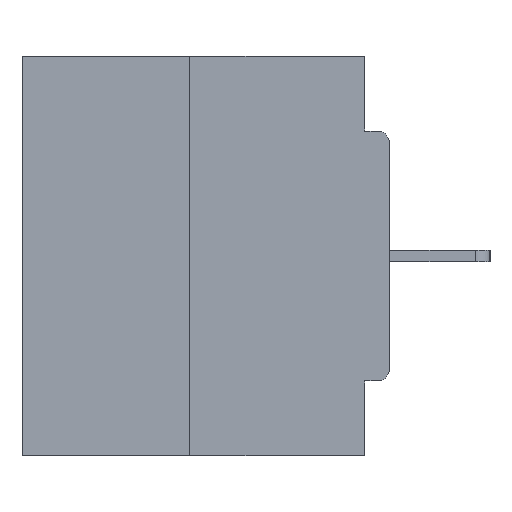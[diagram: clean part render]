
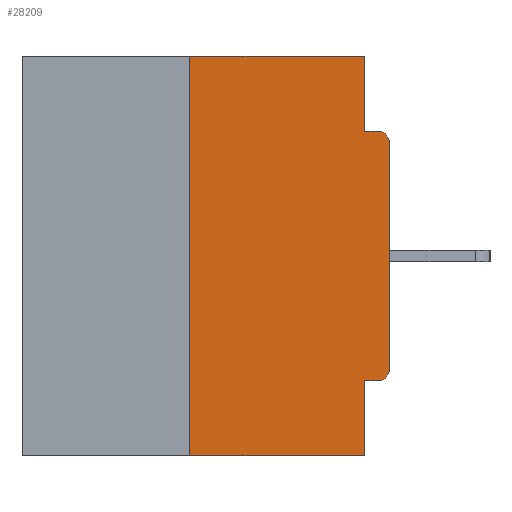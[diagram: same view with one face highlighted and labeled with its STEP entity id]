
A CAD part, left-side view. The second image highlights one B-rep face of the part: STEP entity #28209.
In plain terms, the highlighted planar face has unit normal (-1, 0, 0).
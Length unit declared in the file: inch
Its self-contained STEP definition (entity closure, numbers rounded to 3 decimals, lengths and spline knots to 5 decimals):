
#56 = VERTEX_POINT ( 'NONE', #19696 ) ;
#76 = EDGE_CURVE ( 'NONE', #7154, #5637, #4236, .T. ) ;
#476 = CARTESIAN_POINT ( 'NONE',  ( 0., 0.031, -0.5 ) ) ;
#737 = VERTEX_POINT ( 'NONE', #1125 ) ;
#1125 = CARTESIAN_POINT ( 'NONE',  ( 0., 0., -0.1085 ) ) ;
#2009 = CARTESIAN_POINT ( 'NONE',  ( 0., 0., 0. ) ) ;
#2013 = EDGE_CURVE ( 'NONE', #7154, #56, #16292, .T. ) ;
#2157 = CARTESIAN_POINT ( 'NONE',  ( 0., 0., -0.3915 ) ) ;
#2371 = VECTOR ( 'NONE', #6796, 39.37008 ) ;
#2433 = CARTESIAN_POINT ( 'NONE',  ( 0., 0.031, 0. ) ) ;
#2500 = CARTESIAN_POINT ( 'NONE',  ( 0., 0.25, -0.5 ) ) ;
#2598 = EDGE_CURVE ( 'NONE', #9796, #28735, #20924, .T. ) ;
#3002 = VECTOR ( 'NONE', #19930, 39.37008 ) ;
#3022 = VERTEX_POINT ( 'NONE', #10554 ) ;
#3352 = VECTOR ( 'NONE', #7862, 39.37008 ) ;
#3403 = ORIENTED_EDGE ( 'NONE', *, *, #21245, .F. ) ;
#4236 = LINE ( 'NONE', #9929, #3352 ) ;
#5213 = ORIENTED_EDGE ( 'NONE', *, *, #33166, .F. ) ;
#5637 = VERTEX_POINT ( 'NONE', #30311 ) ;
#5717 = CARTESIAN_POINT ( 'NONE',  ( 0., 0.46, 0. ) ) ;
#6022 = VECTOR ( 'NONE', #21769, 39.37008 ) ;
#6678 = PLANE ( 'NONE',  #7791 ) ;
#6796 = DIRECTION ( 'NONE',  ( 0., 0., 1. ) ) ;
#6994 = CARTESIAN_POINT ( 'NONE',  ( 0., 0.25, 0. ) ) ;
#7154 = VERTEX_POINT ( 'NONE', #2500 ) ;
#7791 = AXIS2_PLACEMENT_3D ( 'NONE', #33736, #25744, #9480 ) ;
#7862 = DIRECTION ( 'NONE',  ( 0., -1., 0. ) ) ;
#9480 = DIRECTION ( 'NONE',  ( 0., 0., -1. ) ) ;
#9796 = VERTEX_POINT ( 'NONE', #30567 ) ;
#9929 = CARTESIAN_POINT ( 'NONE',  ( 0., 0.46, -0.5 ) ) ;
#10049 = ORIENTED_EDGE ( 'NONE', *, *, #25819, .F. ) ;
#10422 = DIRECTION ( 'NONE',  ( 0., 0., 1. ) ) ;
#10554 = CARTESIAN_POINT ( 'NONE',  ( 0., 0.031, -0.4065 ) ) ;
#10928 = CIRCLE ( 'NONE', #29133, 0.015 ) ;
#10967 = LINE ( 'NONE', #5717, #24547 ) ;
#11177 = DIRECTION ( 'NONE',  ( 0., -1., 0. ) ) ;
#11212 = EDGE_LOOP ( 'NONE', ( #5213, #28660, #30343, #34563, #10049, #19024, #35021, #14332, #16403, #3403 ) ) ;
#13380 = LINE ( 'NONE', #2433, #6022 ) ;
#13396 = DIRECTION ( 'NONE',  ( 0., 1., 0. ) ) ;
#13629 = VECTOR ( 'NONE', #13396, 39.37008 ) ;
#14332 = ORIENTED_EDGE ( 'NONE', *, *, #22462, .T. ) ;
#14371 = CARTESIAN_POINT ( 'NONE',  ( 0., 0.015, -0.0935 ) ) ;
#14601 = CARTESIAN_POINT ( 'NONE',  ( 0., 0.015, -0.1085 ) ) ;
#15826 = CIRCLE ( 'NONE', #17992, 0.015 ) ;
#15875 = CARTESIAN_POINT ( 'NONE',  ( 0., 0.015, -0.3915 ) ) ;
#16292 = LINE ( 'NONE', #6994, #2371 ) ;
#16318 = EDGE_CURVE ( 'NONE', #20680, #16497, #10928, .T. ) ;
#16403 = ORIENTED_EDGE ( 'NONE', *, *, #2598, .F. ) ;
#16497 = VERTEX_POINT ( 'NONE', #2157 ) ;
#16504 = CARTESIAN_POINT ( 'NONE',  ( 0., 0., -0.0935 ) ) ;
#16627 = DIRECTION ( 'NONE',  ( 0., -1., 0. ) ) ;
#17295 = VERTEX_POINT ( 'NONE', #22273 ) ;
#17339 = DIRECTION ( 'NONE',  ( 0., 0., -1. ) ) ;
#17687 = FACE_OUTER_BOUND ( 'NONE', #11212, .T. ) ;
#17992 = AXIS2_PLACEMENT_3D ( 'NONE', #14601, #33455, #17339 ) ;
#18635 = DIRECTION ( 'NONE',  ( 0., 0., -1. ) ) ;
#19024 = ORIENTED_EDGE ( 'NONE', *, *, #16318, .T. ) ;
#19696 = CARTESIAN_POINT ( 'NONE',  ( 0., 0.25, 0. ) ) ;
#19930 = DIRECTION ( 'NONE',  ( 0., 0., -1. ) ) ;
#20680 = VERTEX_POINT ( 'NONE', #30007 ) ;
#20924 = LINE ( 'NONE', #16504, #34377 ) ;
#21245 = EDGE_CURVE ( 'NONE', #17295, #9796, #13380, .T. ) ;
#21769 = DIRECTION ( 'NONE',  ( 0., 0., -1. ) ) ;
#22273 = CARTESIAN_POINT ( 'NONE',  ( 0., 0.031, 0. ) ) ;
#22462 = EDGE_CURVE ( 'NONE', #737, #28735, #15826, .T. ) ;
#24512 = EDGE_CURVE ( 'NONE', #16497, #737, #25027, .T. ) ;
#24547 = VECTOR ( 'NONE', #11177, 39.37008 ) ;
#25027 = LINE ( 'NONE', #2009, #32160 ) ;
#25744 = DIRECTION ( 'NONE',  ( 1., 0., 0. ) ) ;
#25819 = EDGE_CURVE ( 'NONE', #20680, #3022, #27153, .T. ) ;
#27153 = LINE ( 'NONE', #29578, #13629 ) ;
#28209 = ADVANCED_FACE ( 'NONE', ( #17687 ), #6678, .F. ) ;
#28660 = ORIENTED_EDGE ( 'NONE', *, *, #2013, .F. ) ;
#28735 = VERTEX_POINT ( 'NONE', #14371 ) ;
#29133 = AXIS2_PLACEMENT_3D ( 'NONE', #15875, #34744, #18635 ) ;
#29578 = CARTESIAN_POINT ( 'NONE',  ( 0., 0., -0.4065 ) ) ;
#30007 = CARTESIAN_POINT ( 'NONE',  ( 0., 0.015, -0.4065 ) ) ;
#30311 = CARTESIAN_POINT ( 'NONE',  ( 0., 0.031, -0.5 ) ) ;
#30343 = ORIENTED_EDGE ( 'NONE', *, *, #76, .T. ) ;
#30567 = CARTESIAN_POINT ( 'NONE',  ( 0., 0.031, -0.0935 ) ) ;
#31198 = LINE ( 'NONE', #476, #3002 ) ;
#32160 = VECTOR ( 'NONE', #10422, 39.37008 ) ;
#33166 = EDGE_CURVE ( 'NONE', #56, #17295, #10967, .T. ) ;
#33455 = DIRECTION ( 'NONE',  ( -1., 0., 0. ) ) ;
#33736 = CARTESIAN_POINT ( 'NONE',  ( 0., 0.46, 0. ) ) ;
#33841 = EDGE_CURVE ( 'NONE', #3022, #5637, #31198, .T. ) ;
#34377 = VECTOR ( 'NONE', #16627, 39.37008 ) ;
#34563 = ORIENTED_EDGE ( 'NONE', *, *, #33841, .F. ) ;
#34744 = DIRECTION ( 'NONE',  ( -1., 0., 0. ) ) ;
#35021 = ORIENTED_EDGE ( 'NONE', *, *, #24512, .T. ) ;
